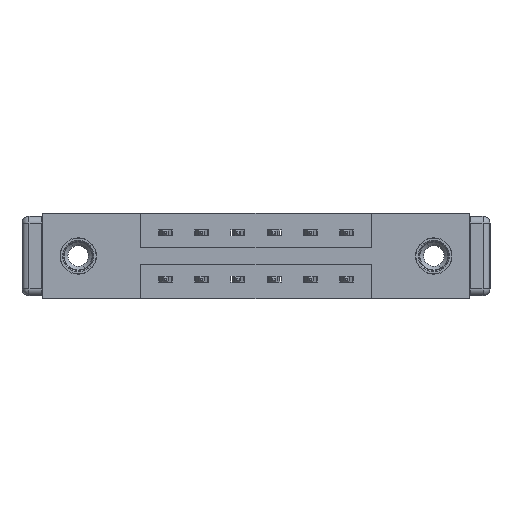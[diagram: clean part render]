
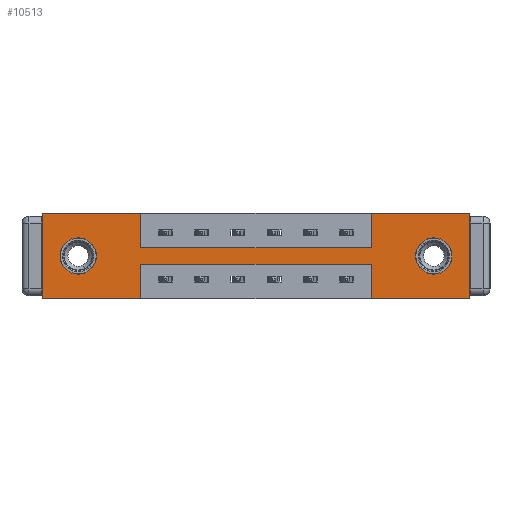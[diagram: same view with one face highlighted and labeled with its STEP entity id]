
A CAD part, front view. The second image highlights one B-rep face of the part: STEP entity #10513.
In plain terms, the highlighted planar face has unit normal (0, -1, 0).
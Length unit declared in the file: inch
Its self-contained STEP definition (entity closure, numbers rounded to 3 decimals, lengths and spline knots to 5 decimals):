
#24 = CARTESIAN_POINT ( 'NONE',  ( 0.425, 0., 0. ) ) ;
#156 = LINE ( 'NONE', #9918, #732 ) ;
#171 = EDGE_CURVE ( 'NONE', #9065, #5981, #354, .T. ) ;
#239 = VECTOR ( 'NONE', #6264, 39.37008 ) ;
#354 = LINE ( 'NONE', #8192, #3389 ) ;
#383 = ORIENTED_EDGE ( 'NONE', *, *, #3653, .T. ) ;
#412 = EDGE_LOOP ( 'NONE', ( #7977, #11788, #6094, #9346, #4041, #3991, #3131, #7865, #1695, #8178, #4030, #10288 ) ) ;
#439 = DIRECTION ( 'NONE',  ( -1., 0., 0. ) ) ;
#695 = DIRECTION ( 'NONE',  ( 1., 0., 0. ) ) ;
#732 = VECTOR ( 'NONE', #7288, 39.37008 ) ;
#742 = AXIS2_PLACEMENT_3D ( 'NONE', #9730, #3168, #4981 ) ;
#892 = DIRECTION ( 'NONE',  ( 0., 0., 1. ) ) ;
#919 = CARTESIAN_POINT ( 'NONE',  ( 1.842, 0., 0. ) ) ;
#1123 = EDGE_CURVE ( 'NONE', #8151, #3962, #4324, .T. ) ;
#1301 = CARTESIAN_POINT ( 'NONE',  ( 1.687, 0., -0.107 ) ) ;
#1342 = EDGE_CURVE ( 'NONE', #10198, #7230, #8865, .T. ) ;
#1411 = CARTESIAN_POINT ( 'NONE',  ( 0.155, 0., -0.185 ) ) ;
#1419 = CARTESIAN_POINT ( 'NONE',  ( 0.425, 0., -0.37 ) ) ;
#1425 = CARTESIAN_POINT ( 'NONE',  ( 1.842, 0., -0.37 ) ) ;
#1518 = DIRECTION ( 'NONE',  ( 0., 1., 0. ) ) ;
#1545 = DIRECTION ( 'NONE',  ( 0., -1., 0. ) ) ;
#1676 = DIRECTION ( 'NONE',  ( 0., 0., -1. ) ) ;
#1695 = ORIENTED_EDGE ( 'NONE', *, *, #6145, .F. ) ;
#1715 = FACE_BOUND ( 'NONE', #9736, .T. ) ;
#1828 = ORIENTED_EDGE ( 'NONE', *, *, #4167, .T. ) ;
#1860 = VECTOR ( 'NONE', #695, 39.37008 ) ;
#1995 = VERTEX_POINT ( 'NONE', #5029 ) ;
#2116 = CARTESIAN_POINT ( 'NONE',  ( 1.417, 0., 0. ) ) ;
#2130 = VECTOR ( 'NONE', #2774, 39.37008 ) ;
#2145 = AXIS2_PLACEMENT_3D ( 'NONE', #7925, #9742, #3178 ) ;
#2227 = VERTEX_POINT ( 'NONE', #10116 ) ;
#2420 = CARTESIAN_POINT ( 'NONE',  ( 0., 0., 0. ) ) ;
#2449 = VERTEX_POINT ( 'NONE', #2488 ) ;
#2488 = CARTESIAN_POINT ( 'NONE',  ( 1.687, 0., -0.263 ) ) ;
#2660 = LINE ( 'NONE', #7955, #3689 ) ;
#2774 = DIRECTION ( 'NONE',  ( 0., 0., -1. ) ) ;
#2862 = CIRCLE ( 'NONE', #2145, 0.078 ) ;
#2867 = CARTESIAN_POINT ( 'NONE',  ( 1.417, 0., 0. ) ) ;
#2868 = DIRECTION ( 'NONE',  ( 1., 0., 0. ) ) ;
#3131 = ORIENTED_EDGE ( 'NONE', *, *, #9130, .F. ) ;
#3168 = DIRECTION ( 'NONE',  ( 0., 1., 0. ) ) ;
#3178 = DIRECTION ( 'NONE',  ( 0., 0., -1. ) ) ;
#3389 = VECTOR ( 'NONE', #1676, 39.37008 ) ;
#3469 = AXIS2_PLACEMENT_3D ( 'NONE', #1411, #1518, #4307 ) ;
#3475 = CARTESIAN_POINT ( 'NONE',  ( 0.155, 0., -0.107 ) ) ;
#3653 = EDGE_CURVE ( 'NONE', #6010, #2449, #2862, .T. ) ;
#3689 = VECTOR ( 'NONE', #439, 39.37008 ) ;
#3804 = VECTOR ( 'NONE', #7371, 39.37008 ) ;
#3962 = VERTEX_POINT ( 'NONE', #3475 ) ;
#3991 = ORIENTED_EDGE ( 'NONE', *, *, #10919, .F. ) ;
#4030 = ORIENTED_EDGE ( 'NONE', *, *, #1342, .F. ) ;
#4041 = ORIENTED_EDGE ( 'NONE', *, *, #11556, .F. ) ;
#4134 = CIRCLE ( 'NONE', #11328, 0.078 ) ;
#4167 = EDGE_CURVE ( 'NONE', #2449, #6010, #7212, .T. ) ;
#4183 = EDGE_CURVE ( 'NONE', #2227, #9065, #9990, .T. ) ;
#4189 = VERTEX_POINT ( 'NONE', #1425 ) ;
#4223 = FACE_BOUND ( 'NONE', #6528, .T. ) ;
#4242 = CARTESIAN_POINT ( 'NONE',  ( 0.425, 0., 0. ) ) ;
#4307 = DIRECTION ( 'NONE',  ( 0., 0., 1. ) ) ;
#4324 = CIRCLE ( 'NONE', #3469, 0.078 ) ;
#4432 = EDGE_CURVE ( 'NONE', #5981, #10198, #2660, .T. ) ;
#4737 = CARTESIAN_POINT ( 'NONE',  ( 0., 0., 0. ) ) ;
#4809 = LINE ( 'NONE', #5311, #1860 ) ;
#4981 = DIRECTION ( 'NONE',  ( 0., 0., -1. ) ) ;
#5029 = CARTESIAN_POINT ( 'NONE',  ( 1.417, 0., -0.15 ) ) ;
#5113 = EDGE_CURVE ( 'NONE', #3962, #8151, #4134, .T. ) ;
#5311 = CARTESIAN_POINT ( 'NONE',  ( 0., 0., 0. ) ) ;
#5572 = CARTESIAN_POINT ( 'NONE',  ( 1.417, 0., -0.37 ) ) ;
#5879 = VECTOR ( 'NONE', #6152, 39.37008 ) ;
#5981 = VERTEX_POINT ( 'NONE', #1419 ) ;
#6002 = CARTESIAN_POINT ( 'NONE',  ( 0.425, 0., -0.15 ) ) ;
#6010 = VERTEX_POINT ( 'NONE', #1301 ) ;
#6094 = ORIENTED_EDGE ( 'NONE', *, *, #9041, .F. ) ;
#6145 = EDGE_CURVE ( 'NONE', #11200, #9379, #11282, .T. ) ;
#6152 = DIRECTION ( 'NONE',  ( 0., 0., 1. ) ) ;
#6264 = DIRECTION ( 'NONE',  ( 0., 0., 1. ) ) ;
#6292 = LINE ( 'NONE', #2867, #7598 ) ;
#6430 = VERTEX_POINT ( 'NONE', #5572 ) ;
#6528 = EDGE_LOOP ( 'NONE', ( #7525, #8486 ) ) ;
#6733 = VERTEX_POINT ( 'NONE', #2116 ) ;
#6815 = LINE ( 'NONE', #919, #2130 ) ;
#7026 = PLANE ( 'NONE',  #7691 ) ;
#7212 = CIRCLE ( 'NONE', #742, 0.078 ) ;
#7230 = VERTEX_POINT ( 'NONE', #2420 ) ;
#7288 = DIRECTION ( 'NONE',  ( -1., 0., 0. ) ) ;
#7306 = CARTESIAN_POINT ( 'NONE',  ( 0., 0., -0.37 ) ) ;
#7371 = DIRECTION ( 'NONE',  ( 0., 0., -1. ) ) ;
#7514 = CARTESIAN_POINT ( 'NONE',  ( 0.155, 0., -0.263 ) ) ;
#7525 = ORIENTED_EDGE ( 'NONE', *, *, #5113, .T. ) ;
#7578 = DIRECTION ( 'NONE',  ( 0., 0., 1. ) ) ;
#7598 = VECTOR ( 'NONE', #7578, 39.37008 ) ;
#7691 = AXIS2_PLACEMENT_3D ( 'NONE', #8793, #1545, #8095 ) ;
#7865 = ORIENTED_EDGE ( 'NONE', *, *, #9358, .F. ) ;
#7912 = DIRECTION ( 'NONE',  ( 1., 0., 0. ) ) ;
#7925 = CARTESIAN_POINT ( 'NONE',  ( 1.687, 0., -0.185 ) ) ;
#7955 = CARTESIAN_POINT ( 'NONE',  ( 0., 0., -0.37 ) ) ;
#7977 = ORIENTED_EDGE ( 'NONE', *, *, #171, .F. ) ;
#7994 = CARTESIAN_POINT ( 'NONE',  ( 1.417, 0., -0.37 ) ) ;
#8095 = DIRECTION ( 'NONE',  ( 0., 0., -1. ) ) ;
#8101 = VERTEX_POINT ( 'NONE', #9270 ) ;
#8151 = VERTEX_POINT ( 'NONE', #7514 ) ;
#8178 = ORIENTED_EDGE ( 'NONE', *, *, #10628, .F. ) ;
#8192 = CARTESIAN_POINT ( 'NONE',  ( 0.425, 0., -0.37 ) ) ;
#8311 = FACE_OUTER_BOUND ( 'NONE', #412, .T. ) ;
#8486 = ORIENTED_EDGE ( 'NONE', *, *, #1123, .T. ) ;
#8745 = DIRECTION ( 'NONE',  ( -1., 0., 0. ) ) ;
#8793 = CARTESIAN_POINT ( 'NONE',  ( 0., 0., -0.37 ) ) ;
#8865 = LINE ( 'NONE', #10180, #239 ) ;
#9031 = CARTESIAN_POINT ( 'NONE',  ( 0.425, 0., -0.15 ) ) ;
#9041 = EDGE_CURVE ( 'NONE', #6430, #2227, #10827, .T. ) ;
#9065 = VERTEX_POINT ( 'NONE', #9518 ) ;
#9130 = EDGE_CURVE ( 'NONE', #1995, #6733, #6292, .T. ) ;
#9270 = CARTESIAN_POINT ( 'NONE',  ( 1.842, 0., 0. ) ) ;
#9293 = VECTOR ( 'NONE', #8745, 39.37008 ) ;
#9346 = ORIENTED_EDGE ( 'NONE', *, *, #9472, .F. ) ;
#9358 = EDGE_CURVE ( 'NONE', #9379, #1995, #10382, .T. ) ;
#9379 = VERTEX_POINT ( 'NONE', #9031 ) ;
#9472 = EDGE_CURVE ( 'NONE', #4189, #6430, #156, .T. ) ;
#9518 = CARTESIAN_POINT ( 'NONE',  ( 0.425, 0., -0.22 ) ) ;
#9601 = LINE ( 'NONE', #4737, #10935 ) ;
#9730 = CARTESIAN_POINT ( 'NONE',  ( 1.687, 0., -0.185 ) ) ;
#9736 = EDGE_LOOP ( 'NONE', ( #383, #1828 ) ) ;
#9742 = DIRECTION ( 'NONE',  ( 0., 1., 0. ) ) ;
#9918 = CARTESIAN_POINT ( 'NONE',  ( 0., 0., -0.37 ) ) ;
#9990 = LINE ( 'NONE', #10737, #9293 ) ;
#10116 = CARTESIAN_POINT ( 'NONE',  ( 1.417, 0., -0.22 ) ) ;
#10180 = CARTESIAN_POINT ( 'NONE',  ( 0., 0., 0. ) ) ;
#10198 = VERTEX_POINT ( 'NONE', #7306 ) ;
#10288 = ORIENTED_EDGE ( 'NONE', *, *, #4432, .F. ) ;
#10382 = LINE ( 'NONE', #6002, #11726 ) ;
#10513 = ADVANCED_FACE ( 'NONE', ( #1715, #4223, #8311 ), #7026, .T. ) ;
#10628 = EDGE_CURVE ( 'NONE', #7230, #11200, #4809, .T. ) ;
#10737 = CARTESIAN_POINT ( 'NONE',  ( 0.425, 0., -0.22 ) ) ;
#10827 = LINE ( 'NONE', #7994, #5879 ) ;
#10919 = EDGE_CURVE ( 'NONE', #6733, #8101, #9601, .T. ) ;
#10935 = VECTOR ( 'NONE', #2868, 39.37008 ) ;
#11074 = DIRECTION ( 'NONE',  ( 0., 1., 0. ) ) ;
#11200 = VERTEX_POINT ( 'NONE', #4242 ) ;
#11282 = LINE ( 'NONE', #24, #3804 ) ;
#11328 = AXIS2_PLACEMENT_3D ( 'NONE', #11986, #11074, #892 ) ;
#11556 = EDGE_CURVE ( 'NONE', #8101, #4189, #6815, .T. ) ;
#11726 = VECTOR ( 'NONE', #7912, 39.37008 ) ;
#11788 = ORIENTED_EDGE ( 'NONE', *, *, #4183, .F. ) ;
#11986 = CARTESIAN_POINT ( 'NONE',  ( 0.155, 0., -0.185 ) ) ;
